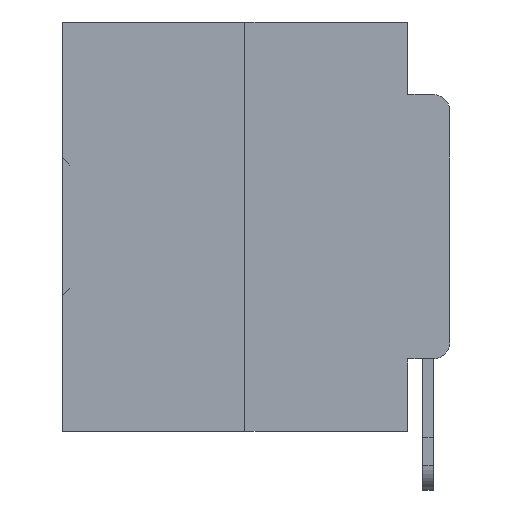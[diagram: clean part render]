
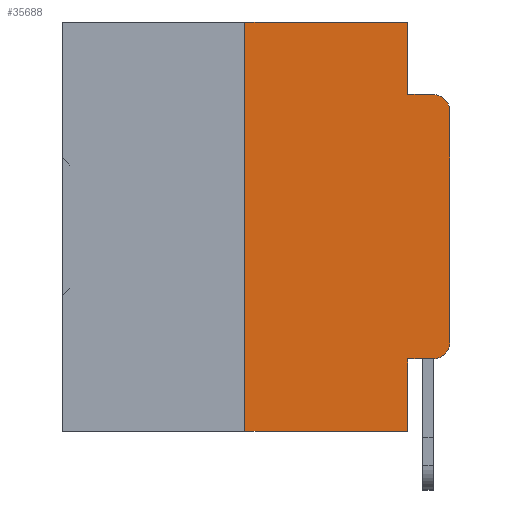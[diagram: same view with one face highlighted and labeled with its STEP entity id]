
A CAD part, left-side view. The second image highlights one B-rep face of the part: STEP entity #35688.
In plain terms, the highlighted planar face has unit normal (-1, 0, 0).
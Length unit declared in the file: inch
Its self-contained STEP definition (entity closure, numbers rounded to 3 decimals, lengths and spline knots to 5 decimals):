
#316 = CARTESIAN_POINT ( 'NONE',  ( 0., 0.473, -0.5 ) ) ;
#317 = DIRECTION ( 'NONE',  ( 0., 0., -1. ) ) ;
#889 = ORIENTED_EDGE ( 'NONE', *, *, #28091, .F. ) ;
#1350 = ORIENTED_EDGE ( 'NONE', *, *, #3237, .T. ) ;
#2122 = ORIENTED_EDGE ( 'NONE', *, *, #8527, .T. ) ;
#2548 = ORIENTED_EDGE ( 'NONE', *, *, #21894, .T. ) ;
#2712 = VERTEX_POINT ( 'NONE', #19334 ) ;
#2732 = CARTESIAN_POINT ( 'NONE',  ( 0., 0., -0.1085 ) ) ;
#2735 = CIRCLE ( 'NONE', #32777, 0.02 ) ;
#2999 = LINE ( 'NONE', #29985, #9981 ) ;
#3237 = EDGE_CURVE ( 'NONE', #19149, #10428, #2999, .T. ) ;
#3311 = ORIENTED_EDGE ( 'NONE', *, *, #23697, .F. ) ;
#3457 = DIRECTION ( 'NONE',  ( 0., -1., 0. ) ) ;
#3755 = ORIENTED_EDGE ( 'NONE', *, *, #9935, .T. ) ;
#3927 = ORIENTED_EDGE ( 'NONE', *, *, #18482, .F. ) ;
#3939 = CARTESIAN_POINT ( 'NONE',  ( 0., 0.25, 0. ) ) ;
#4449 = DIRECTION ( 'NONE',  ( -1., 0., 0. ) ) ;
#4649 = CARTESIAN_POINT ( 'NONE',  ( 0., 0.051, 0. ) ) ;
#4792 = EDGE_CURVE ( 'NONE', #10635, #19307, #26893, .T. ) ;
#6385 = VERTEX_POINT ( 'NONE', #33975 ) ;
#6872 = ORIENTED_EDGE ( 'NONE', *, *, #4792, .F. ) ;
#6874 = CARTESIAN_POINT ( 'NONE',  ( 0., 0.051, -0.4115 ) ) ;
#6935 = CARTESIAN_POINT ( 'NONE',  ( 0., 0.051, -0.0885 ) ) ;
#8255 = VERTEX_POINT ( 'NONE', #22848 ) ;
#8406 = VERTEX_POINT ( 'NONE', #26169 ) ;
#8527 = EDGE_CURVE ( 'NONE', #8255, #10415, #11185, .T. ) ;
#9367 = VECTOR ( 'NONE', #20609, 39.37008 ) ;
#9935 = EDGE_CURVE ( 'NONE', #10428, #8255, #2735, .T. ) ;
#9981 = VECTOR ( 'NONE', #35469, 39.37008 ) ;
#10415 = VERTEX_POINT ( 'NONE', #2732 ) ;
#10421 = CARTESIAN_POINT ( 'NONE',  ( 0., 0.473, 0. ) ) ;
#10428 = VERTEX_POINT ( 'NONE', #14560 ) ;
#10635 = VERTEX_POINT ( 'NONE', #3939 ) ;
#10688 = VERTEX_POINT ( 'NONE', #27239 ) ;
#11185 = LINE ( 'NONE', #12099, #18834 ) ;
#11762 = VECTOR ( 'NONE', #31545, 39.37008 ) ;
#11804 = EDGE_LOOP ( 'NONE', ( #2122, #2548, #3311, #3927, #6872, #26167, #12898, #889, #1350, #3755 ) ) ;
#12099 = CARTESIAN_POINT ( 'NONE',  ( 0., 0., 0. ) ) ;
#12620 = CARTESIAN_POINT ( 'NONE',  ( 0., 0.051, 0. ) ) ;
#12898 = ORIENTED_EDGE ( 'NONE', *, *, #27523, .T. ) ;
#14426 = CARTESIAN_POINT ( 'NONE',  ( 0., 0.473, 0. ) ) ;
#14552 = DIRECTION ( 'NONE',  ( 1., 0., 0. ) ) ;
#14560 = CARTESIAN_POINT ( 'NONE',  ( 0., 0.02, -0.4115 ) ) ;
#15526 = DIRECTION ( 'NONE',  ( 0., 0., -1. ) ) ;
#18042 = DIRECTION ( 'NONE',  ( -1., 0., 0. ) ) ;
#18482 = EDGE_CURVE ( 'NONE', #19307, #6385, #27909, .T. ) ;
#18521 = VECTOR ( 'NONE', #21967, 39.37008 ) ;
#18834 = VECTOR ( 'NONE', #34656, 39.37008 ) ;
#19149 = VERTEX_POINT ( 'NONE', #6874 ) ;
#19307 = VERTEX_POINT ( 'NONE', #4649 ) ;
#19334 = CARTESIAN_POINT ( 'NONE',  ( 0., 0.25, -0.5 ) ) ;
#20609 = DIRECTION ( 'NONE',  ( 0., 0., -1. ) ) ;
#21312 = AXIS2_PLACEMENT_3D ( 'NONE', #14426, #14552, #34175 ) ;
#21835 = CARTESIAN_POINT ( 'NONE',  ( 0., 0.02, -0.1085 ) ) ;
#21894 = EDGE_CURVE ( 'NONE', #10415, #8406, #34666, .T. ) ;
#21967 = DIRECTION ( 'NONE',  ( 0., -1., 0. ) ) ;
#22450 = LINE ( 'NONE', #316, #36412 ) ;
#22848 = CARTESIAN_POINT ( 'NONE',  ( 0., 0., -0.3915 ) ) ;
#23697 = EDGE_CURVE ( 'NONE', #6385, #8406, #33990, .T. ) ;
#24638 = DIRECTION ( 'NONE',  ( 0., 0., -1. ) ) ;
#25749 = PLANE ( 'NONE',  #21312 ) ;
#25927 = CARTESIAN_POINT ( 'NONE',  ( 0., 0.25, 0. ) ) ;
#26167 = ORIENTED_EDGE ( 'NONE', *, *, #27426, .F. ) ;
#26169 = CARTESIAN_POINT ( 'NONE',  ( 0., 0.02, -0.0885 ) ) ;
#26893 = LINE ( 'NONE', #10421, #18521 ) ;
#27239 = CARTESIAN_POINT ( 'NONE',  ( 0., 0.051, -0.5 ) ) ;
#27426 = EDGE_CURVE ( 'NONE', #2712, #10635, #34267, .T. ) ;
#27458 = VECTOR ( 'NONE', #32488, 39.37008 ) ;
#27523 = EDGE_CURVE ( 'NONE', #2712, #10688, #22450, .T. ) ;
#27909 = LINE ( 'NONE', #12620, #34451 ) ;
#28091 = EDGE_CURVE ( 'NONE', #19149, #10688, #32034, .T. ) ;
#29296 = AXIS2_PLACEMENT_3D ( 'NONE', #21835, #4449, #24638 ) ;
#29985 = CARTESIAN_POINT ( 'NONE',  ( 0., 0.051, -0.4115 ) ) ;
#31545 = DIRECTION ( 'NONE',  ( 0., 0., 1. ) ) ;
#31864 = CARTESIAN_POINT ( 'NONE',  ( 0., 0.051, 0. ) ) ;
#32034 = LINE ( 'NONE', #31864, #9367 ) ;
#32488 = DIRECTION ( 'NONE',  ( 0., -1., 0. ) ) ;
#32777 = AXIS2_PLACEMENT_3D ( 'NONE', #34846, #18042, #317 ) ;
#33975 = CARTESIAN_POINT ( 'NONE',  ( 0., 0.051, -0.0885 ) ) ;
#33990 = LINE ( 'NONE', #6935, #27458 ) ;
#34175 = DIRECTION ( 'NONE',  ( 0., 0., -1. ) ) ;
#34267 = LINE ( 'NONE', #25927, #11762 ) ;
#34451 = VECTOR ( 'NONE', #15526, 39.37008 ) ;
#34656 = DIRECTION ( 'NONE',  ( 0., 0., 1. ) ) ;
#34666 = CIRCLE ( 'NONE', #29296, 0.02 ) ;
#34846 = CARTESIAN_POINT ( 'NONE',  ( 0., 0.02, -0.3915 ) ) ;
#35460 = FACE_OUTER_BOUND ( 'NONE', #11804, .T. ) ;
#35469 = DIRECTION ( 'NONE',  ( 0., -1., 0. ) ) ;
#35688 = ADVANCED_FACE ( 'NONE', ( #35460 ), #25749, .F. ) ;
#36412 = VECTOR ( 'NONE', #3457, 39.37008 ) ;
